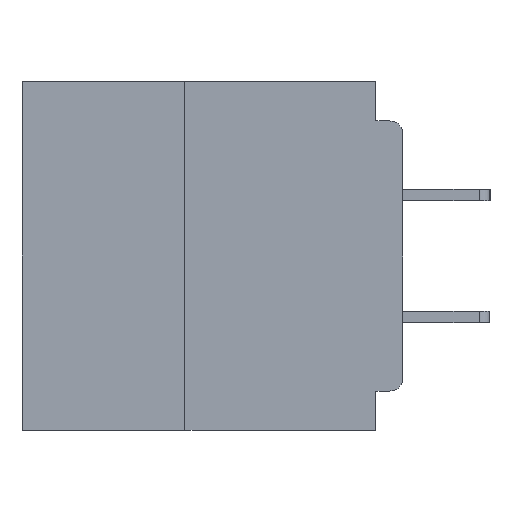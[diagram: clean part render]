
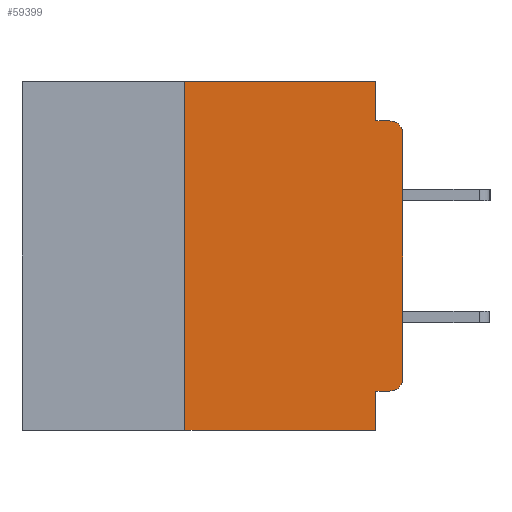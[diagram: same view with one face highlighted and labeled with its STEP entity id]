
A CAD part, left-side view. The second image highlights one B-rep face of the part: STEP entity #59399.
In plain terms, the highlighted planar face has unit normal (-1, 0, 0).
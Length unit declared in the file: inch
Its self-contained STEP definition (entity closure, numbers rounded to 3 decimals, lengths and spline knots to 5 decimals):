
#179 = CARTESIAN_POINT ( 'NONE',  ( 0., 0.031, -0.355 ) ) ;
#1275 = CARTESIAN_POINT ( 'NONE',  ( 0., 0.25, -0.4 ) ) ;
#3713 = CARTESIAN_POINT ( 'NONE',  ( 0., 0.015, -0.355 ) ) ;
#4923 = DIRECTION ( 'NONE',  ( -1., 0., 0. ) ) ;
#5425 = VECTOR ( 'NONE', #14693, 39.37008 ) ;
#6123 = CARTESIAN_POINT ( 'NONE',  ( 0., 0.437, 0. ) ) ;
#6348 = ORIENTED_EDGE ( 'NONE', *, *, #33204, .T. ) ;
#6808 = LINE ( 'NONE', #37356, #44137 ) ;
#8310 = AXIS2_PLACEMENT_3D ( 'NONE', #20019, #54084, #24877 ) ;
#9278 = LINE ( 'NONE', #1275, #59508 ) ;
#9773 = CARTESIAN_POINT ( 'NONE',  ( 0., 0.437, 0. ) ) ;
#9797 = CARTESIAN_POINT ( 'NONE',  ( 0., 0., -0.045 ) ) ;
#10221 = CARTESIAN_POINT ( 'NONE',  ( 0., 0., -0.355 ) ) ;
#11661 = EDGE_CURVE ( 'NONE', #51345, #32541, #43977, .T. ) ;
#12429 = VERTEX_POINT ( 'NONE', #31314 ) ;
#12587 = VERTEX_POINT ( 'NONE', #47910 ) ;
#14184 = DIRECTION ( 'NONE',  ( 0., 0., -1. ) ) ;
#14693 = DIRECTION ( 'NONE',  ( 0., -1., 0. ) ) ;
#15044 = CARTESIAN_POINT ( 'NONE',  ( 0., 0.015, -0.045 ) ) ;
#16242 = FACE_OUTER_BOUND ( 'NONE', #53039, .T. ) ;
#16716 = VERTEX_POINT ( 'NONE', #18984 ) ;
#17405 = VECTOR ( 'NONE', #39022, 39.37008 ) ;
#17924 = DIRECTION ( 'NONE',  ( 0., 0., 1. ) ) ;
#18984 = CARTESIAN_POINT ( 'NONE',  ( 0., 0.031, -0.4 ) ) ;
#19264 = EDGE_CURVE ( 'NONE', #22610, #30058, #57246, .T. ) ;
#19984 = CARTESIAN_POINT ( 'NONE',  ( 0., 0.25, -0.4 ) ) ;
#20019 = CARTESIAN_POINT ( 'NONE',  ( 0., 0.015, -0.06 ) ) ;
#20504 = EDGE_CURVE ( 'NONE', #12587, #12429, #6808, .T. ) ;
#20850 = DIRECTION ( 'NONE',  ( 0., 0., -1. ) ) ;
#22362 = ORIENTED_EDGE ( 'NONE', *, *, #50816, .F. ) ;
#22610 = VERTEX_POINT ( 'NONE', #55349 ) ;
#23268 = EDGE_CURVE ( 'NONE', #37068, #16716, #24777, .T. ) ;
#24777 = LINE ( 'NONE', #35935, #60551 ) ;
#24877 = DIRECTION ( 'NONE',  ( 0., 0., -1. ) ) ;
#25474 = ORIENTED_EDGE ( 'NONE', *, *, #53692, .T. ) ;
#26742 = LINE ( 'NONE', #43336, #52633 ) ;
#29252 = EDGE_CURVE ( 'NONE', #37068, #41620, #9278, .T. ) ;
#30058 = VERTEX_POINT ( 'NONE', #57479 ) ;
#30738 = ORIENTED_EDGE ( 'NONE', *, *, #46251, .F. ) ;
#31314 = CARTESIAN_POINT ( 'NONE',  ( 0., 0., -0.06 ) ) ;
#31379 = ORIENTED_EDGE ( 'NONE', *, *, #42317, .F. ) ;
#32341 = CARTESIAN_POINT ( 'NONE',  ( 0., 0.031, 0. ) ) ;
#32541 = VERTEX_POINT ( 'NONE', #179 ) ;
#33204 = EDGE_CURVE ( 'NONE', #12429, #56526, #54440, .T. ) ;
#33673 = ORIENTED_EDGE ( 'NONE', *, *, #20504, .T. ) ;
#33943 = CARTESIAN_POINT ( 'NONE',  ( 0., 0.25, 0. ) ) ;
#34141 = CARTESIAN_POINT ( 'NONE',  ( 0., 0.015, -0.34 ) ) ;
#35935 = CARTESIAN_POINT ( 'NONE',  ( 0., 0.437, -0.4 ) ) ;
#37068 = VERTEX_POINT ( 'NONE', #19984 ) ;
#37085 = ORIENTED_EDGE ( 'NONE', *, *, #11661, .F. ) ;
#37356 = CARTESIAN_POINT ( 'NONE',  ( 0., 0., 0. ) ) ;
#39022 = DIRECTION ( 'NONE',  ( 0., -1., 0. ) ) ;
#39077 = DIRECTION ( 'NONE',  ( 0., 0., -1. ) ) ;
#39431 = DIRECTION ( 'NONE',  ( 0., 1., 0. ) ) ;
#40588 = AXIS2_PLACEMENT_3D ( 'NONE', #6123, #49989, #20850 ) ;
#40837 = DIRECTION ( 'NONE',  ( 0., -1., 0. ) ) ;
#41620 = VERTEX_POINT ( 'NONE', #33943 ) ;
#42181 = CIRCLE ( 'NONE', #43153, 0.015 ) ;
#42317 = EDGE_CURVE ( 'NONE', #30058, #56526, #56893, .T. ) ;
#42362 = DIRECTION ( 'NONE',  ( 0., 0., -1. ) ) ;
#42454 = VECTOR ( 'NONE', #39431, 39.37008 ) ;
#43153 = AXIS2_PLACEMENT_3D ( 'NONE', #34141, #4923, #39077 ) ;
#43336 = CARTESIAN_POINT ( 'NONE',  ( 0., 0.031, -0.4 ) ) ;
#43977 = LINE ( 'NONE', #10221, #42454 ) ;
#44137 = VECTOR ( 'NONE', #17924, 39.37008 ) ;
#44334 = LINE ( 'NONE', #9773, #5425 ) ;
#45111 = PLANE ( 'NONE',  #40588 ) ;
#46251 = EDGE_CURVE ( 'NONE', #32541, #16716, #26742, .T. ) ;
#47910 = CARTESIAN_POINT ( 'NONE',  ( 0., 0., -0.34 ) ) ;
#48057 = ORIENTED_EDGE ( 'NONE', *, *, #23268, .T. ) ;
#49163 = ORIENTED_EDGE ( 'NONE', *, *, #19264, .F. ) ;
#49989 = DIRECTION ( 'NONE',  ( 1., 0., 0. ) ) ;
#50816 = EDGE_CURVE ( 'NONE', #41620, #22610, #44334, .T. ) ;
#51345 = VERTEX_POINT ( 'NONE', #3713 ) ;
#52633 = VECTOR ( 'NONE', #14184, 39.37008 ) ;
#53039 = EDGE_LOOP ( 'NONE', ( #33673, #6348, #31379, #49163, #22362, #56740, #48057, #30738, #37085, #25474 ) ) ;
#53692 = EDGE_CURVE ( 'NONE', #51345, #12587, #42181, .T. ) ;
#54084 = DIRECTION ( 'NONE',  ( -1., 0., 0. ) ) ;
#54206 = VECTOR ( 'NONE', #42362, 39.37008 ) ;
#54440 = CIRCLE ( 'NONE', #8310, 0.015 ) ;
#55031 = DIRECTION ( 'NONE',  ( 0., 0., 1. ) ) ;
#55349 = CARTESIAN_POINT ( 'NONE',  ( 0., 0.031, 0. ) ) ;
#56526 = VERTEX_POINT ( 'NONE', #15044 ) ;
#56740 = ORIENTED_EDGE ( 'NONE', *, *, #29252, .F. ) ;
#56893 = LINE ( 'NONE', #9797, #17405 ) ;
#57246 = LINE ( 'NONE', #32341, #54206 ) ;
#57479 = CARTESIAN_POINT ( 'NONE',  ( 0., 0.031, -0.045 ) ) ;
#59399 = ADVANCED_FACE ( 'NONE', ( #16242 ), #45111, .F. ) ;
#59508 = VECTOR ( 'NONE', #55031, 39.37008 ) ;
#60551 = VECTOR ( 'NONE', #40837, 39.37008 ) ;
